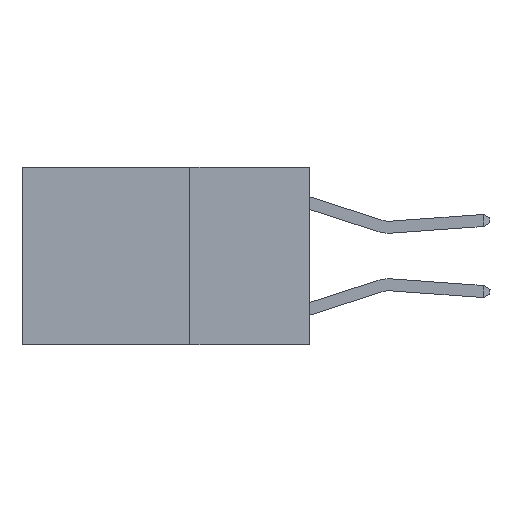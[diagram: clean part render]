
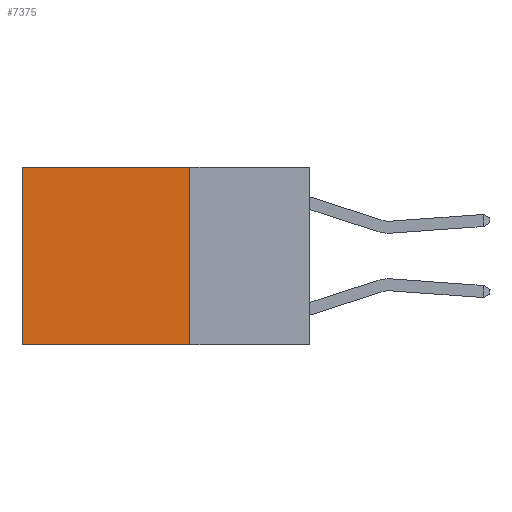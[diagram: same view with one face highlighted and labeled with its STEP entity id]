
A CAD part, left-side view. The second image highlights one B-rep face of the part: STEP entity #7375.
In plain terms, the highlighted planar face has unit normal (-1, 0, 0).
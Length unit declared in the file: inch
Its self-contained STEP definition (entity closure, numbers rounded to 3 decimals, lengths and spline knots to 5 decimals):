
#723 = CARTESIAN_POINT ( 'NONE',  ( 0.2625, 0.25, 0. ) ) ;
#1548 = CARTESIAN_POINT ( 'NONE',  ( 0.2625, 0.25, -0.37 ) ) ;
#1676 = DIRECTION ( 'NONE',  ( 0., 0., -1. ) ) ;
#2207 = DIRECTION ( 'NONE',  ( 0., 0., -1. ) ) ;
#2885 = ORIENTED_EDGE ( 'NONE', *, *, #26068, .F. ) ;
#3511 = CARTESIAN_POINT ( 'NONE',  ( 0.2625, 0.6, 0. ) ) ;
#4105 = DIRECTION ( 'NONE',  ( 1., 0., 0. ) ) ;
#4779 = CARTESIAN_POINT ( 'NONE',  ( 0.2625, 0.6, -0.37 ) ) ;
#5842 = CARTESIAN_POINT ( 'NONE',  ( 0.2625, 0.25, 0. ) ) ;
#6496 = DIRECTION ( 'NONE',  ( 0., 1., 0. ) ) ;
#6534 = FACE_OUTER_BOUND ( 'NONE', #25763, .T. ) ;
#6761 = VECTOR ( 'NONE', #6496, 39.37008 ) ;
#7375 = ADVANCED_FACE ( 'NONE', ( #6534 ), #16794, .F. ) ;
#9475 = ORIENTED_EDGE ( 'NONE', *, *, #12164, .T. ) ;
#9914 = LINE ( 'NONE', #25045, #13979 ) ;
#12023 = DIRECTION ( 'NONE',  ( 0., 1., 0. ) ) ;
#12164 = EDGE_CURVE ( 'NONE', #17270, #14848, #14746, .T. ) ;
#12514 = VERTEX_POINT ( 'NONE', #1548 ) ;
#13979 = VECTOR ( 'NONE', #12023, 39.37008 ) ;
#14746 = LINE ( 'NONE', #24478, #16687 ) ;
#14848 = VERTEX_POINT ( 'NONE', #4779 ) ;
#16099 = AXIS2_PLACEMENT_3D ( 'NONE', #29160, #4105, #1676 ) ;
#16687 = VECTOR ( 'NONE', #2207, 39.37008 ) ;
#16794 = PLANE ( 'NONE',  #16099 ) ;
#17270 = VERTEX_POINT ( 'NONE', #3511 ) ;
#18865 = LINE ( 'NONE', #28803, #6761 ) ;
#20247 = VECTOR ( 'NONE', #30906, 39.37008 ) ;
#22323 = ORIENTED_EDGE ( 'NONE', *, *, #23979, .T. ) ;
#23979 = EDGE_CURVE ( 'NONE', #31869, #17270, #9914, .T. ) ;
#24478 = CARTESIAN_POINT ( 'NONE',  ( 0.2625, 0.6, 0. ) ) ;
#25045 = CARTESIAN_POINT ( 'NONE',  ( 0.2625, 0.25, 0. ) ) ;
#25763 = EDGE_LOOP ( 'NONE', ( #9475, #25847, #2885, #22323 ) ) ;
#25847 = ORIENTED_EDGE ( 'NONE', *, *, #26359, .F. ) ;
#26068 = EDGE_CURVE ( 'NONE', #31869, #12514, #26217, .T. ) ;
#26217 = LINE ( 'NONE', #5842, #20247 ) ;
#26359 = EDGE_CURVE ( 'NONE', #12514, #14848, #18865, .T. ) ;
#28803 = CARTESIAN_POINT ( 'NONE',  ( 0.2625, 0.25, -0.37 ) ) ;
#29160 = CARTESIAN_POINT ( 'NONE',  ( 0.2625, 0.25, 0. ) ) ;
#30906 = DIRECTION ( 'NONE',  ( 0., 0., -1. ) ) ;
#31869 = VERTEX_POINT ( 'NONE', #723 ) ;
